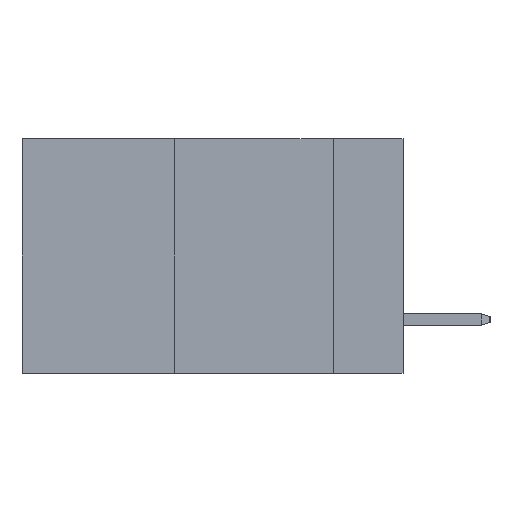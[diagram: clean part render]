
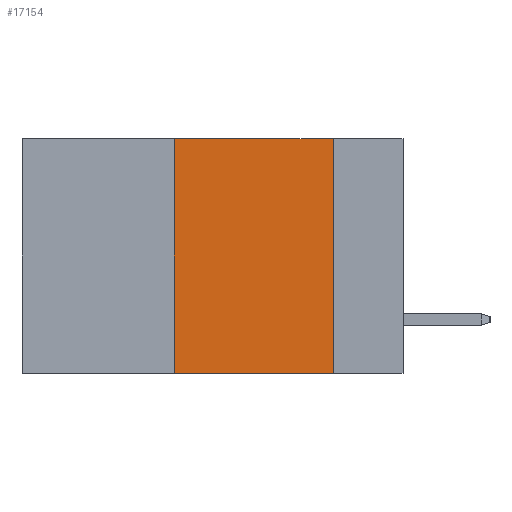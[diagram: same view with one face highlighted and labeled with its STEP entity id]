
A CAD part, left-side view. The second image highlights one B-rep face of the part: STEP entity #17154.
In plain terms, the highlighted planar face has unit normal (-1, 0, 0).
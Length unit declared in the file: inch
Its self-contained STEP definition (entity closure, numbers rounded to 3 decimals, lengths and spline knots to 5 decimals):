
#140 = VERTEX_POINT ( 'NONE', #5931 ) ;
#200 = DIRECTION ( 'NONE',  ( 0., 0., -1. ) ) ;
#406 = CARTESIAN_POINT ( 'NONE',  ( 0., 0.6, 0. ) ) ;
#722 = VECTOR ( 'NONE', #10837, 39.37008 ) ;
#1202 = EDGE_CURVE ( 'NONE', #12525, #3507, #3003, .T. ) ;
#1406 = PLANE ( 'NONE',  #4641 ) ;
#2465 = CARTESIAN_POINT ( 'NONE',  ( 0., 0.6, -0.37 ) ) ;
#2483 = DIRECTION ( 'NONE',  ( 0., 0., -1. ) ) ;
#2580 = CARTESIAN_POINT ( 'NONE',  ( 0., 0.11, 0. ) ) ;
#2664 = ORIENTED_EDGE ( 'NONE', *, *, #11753, .T. ) ;
#2955 = ORIENTED_EDGE ( 'NONE', *, *, #3424, .F. ) ;
#3003 = LINE ( 'NONE', #15499, #6067 ) ;
#3424 = EDGE_CURVE ( 'NONE', #3507, #13287, #5850, .T. ) ;
#3507 = VERTEX_POINT ( 'NONE', #16134 ) ;
#4259 = VECTOR ( 'NONE', #2483, 39.37008 ) ;
#4641 = AXIS2_PLACEMENT_3D ( 'NONE', #7012, #12618, #200 ) ;
#5274 = CARTESIAN_POINT ( 'NONE',  ( 0., 0.36, -0.37 ) ) ;
#5850 = LINE ( 'NONE', #406, #14497 ) ;
#5864 = EDGE_CURVE ( 'NONE', #13287, #140, #15071, .T. ) ;
#5931 = CARTESIAN_POINT ( 'NONE',  ( 0., 0.11, -0.37 ) ) ;
#6051 = ORIENTED_EDGE ( 'NONE', *, *, #1202, .F. ) ;
#6067 = VECTOR ( 'NONE', #11270, 39.37008 ) ;
#7012 = CARTESIAN_POINT ( 'NONE',  ( 0., 0.6, 0. ) ) ;
#7208 = EDGE_LOOP ( 'NONE', ( #8825, #2955, #6051, #2664 ) ) ;
#7600 = CARTESIAN_POINT ( 'NONE',  ( 0., 0.11, 0. ) ) ;
#8205 = FACE_OUTER_BOUND ( 'NONE', #7208, .T. ) ;
#8825 = ORIENTED_EDGE ( 'NONE', *, *, #5864, .F. ) ;
#10837 = DIRECTION ( 'NONE',  ( 0., -1., 0. ) ) ;
#11270 = DIRECTION ( 'NONE',  ( 0., 0., 1. ) ) ;
#11753 = EDGE_CURVE ( 'NONE', #12525, #140, #16620, .T. ) ;
#12525 = VERTEX_POINT ( 'NONE', #5274 ) ;
#12618 = DIRECTION ( 'NONE',  ( 1., 0., 0. ) ) ;
#13287 = VERTEX_POINT ( 'NONE', #7600 ) ;
#14299 = DIRECTION ( 'NONE',  ( 0., -1., 0. ) ) ;
#14497 = VECTOR ( 'NONE', #14299, 39.37008 ) ;
#15071 = LINE ( 'NONE', #2580, #4259 ) ;
#15499 = CARTESIAN_POINT ( 'NONE',  ( 0., 0.36, 0. ) ) ;
#16134 = CARTESIAN_POINT ( 'NONE',  ( 0., 0.36, 0. ) ) ;
#16620 = LINE ( 'NONE', #2465, #722 ) ;
#17154 = ADVANCED_FACE ( 'NONE', ( #8205 ), #1406, .F. ) ;
